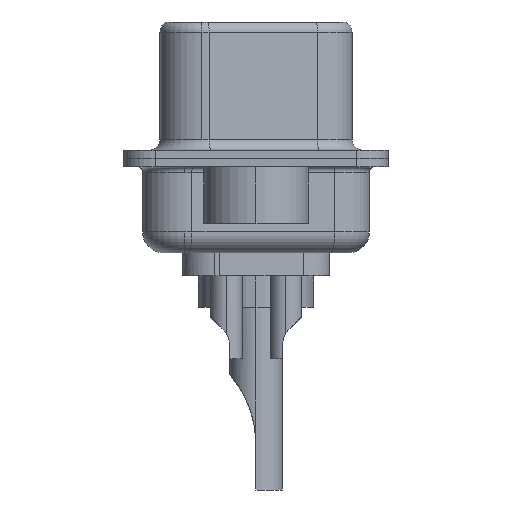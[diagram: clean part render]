
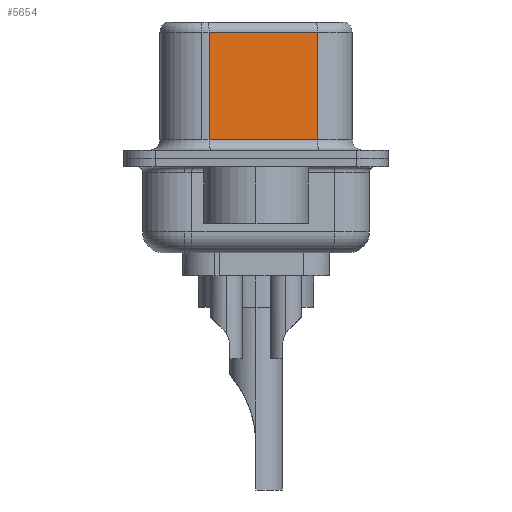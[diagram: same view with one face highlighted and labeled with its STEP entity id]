
A CAD part, left-side view. The second image highlights one B-rep face of the part: STEP entity #5654.
In plain terms, the highlighted planar face has unit normal (-0.985, -0.174, 0).
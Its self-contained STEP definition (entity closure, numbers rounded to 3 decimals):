
#146 = VERTEX_POINT ( 'NONE', #6224 ) ;
#476 = ORIENTED_EDGE ( 'NONE', *, *, #2638, .T. ) ;
#1671 = EDGE_CURVE ( 'NONE', #14607, #146, #11014, .T. ) ;
#1819 = CARTESIAN_POINT ( 'NONE',  ( 4.565, -2.927, 6.52 ) ) ;
#2638 = EDGE_CURVE ( 'NONE', #146, #15769, #15951, .T. ) ;
#3247 = DIRECTION ( 'NONE',  ( -0.174, 0.985, 0. ) ) ;
#3929 = LINE ( 'NONE', #13872, #10312 ) ;
#4091 = CARTESIAN_POINT ( 'NONE',  ( 4.565, -2.927, 0.9 ) ) ;
#4620 = DIRECTION ( 'NONE',  ( 0.174, -0.985, 0. ) ) ;
#5042 = CARTESIAN_POINT ( 'NONE',  ( 4.565, -2.927, 6.02 ) ) ;
#5441 = VECTOR ( 'NONE', #9369, 1000. ) ;
#5654 = ADVANCED_FACE ( 'NONE', ( #14398 ), #15184, .F. ) ;
#6224 = CARTESIAN_POINT ( 'NONE',  ( 3.655, 2.233, 6.02 ) ) ;
#6490 = DIRECTION ( 'NONE',  ( -0.174, 0.985, 0. ) ) ;
#7057 = ORIENTED_EDGE ( 'NONE', *, *, #7170, .F. ) ;
#7162 = LINE ( 'NONE', #16521, #11160 ) ;
#7170 = EDGE_CURVE ( 'NONE', #14607, #16997, #7162, .T. ) ;
#7173 = EDGE_CURVE ( 'NONE', #15769, #16997, #3929, .T. ) ;
#7406 = VECTOR ( 'NONE', #6490, 1000. ) ;
#7483 = ORIENTED_EDGE ( 'NONE', *, *, #1671, .T. ) ;
#8137 = CARTESIAN_POINT ( 'NONE',  ( 3.655, 2.233, 0.9 ) ) ;
#8695 = DIRECTION ( 'NONE',  ( 0., 0., -1. ) ) ;
#9369 = DIRECTION ( 'NONE',  ( 0., 0., -1. ) ) ;
#10312 = VECTOR ( 'NONE', #4620, 1000. ) ;
#10691 = CARTESIAN_POINT ( 'NONE',  ( 4.565, -2.927, 6.02 ) ) ;
#10795 = EDGE_LOOP ( 'NONE', ( #7057, #7483, #476, #11469 ) ) ;
#11014 = LINE ( 'NONE', #5042, #7406 ) ;
#11160 = VECTOR ( 'NONE', #8695, 1000. ) ;
#11429 = DIRECTION ( 'NONE',  ( 0.985, 0.174, 0. ) ) ;
#11469 = ORIENTED_EDGE ( 'NONE', *, *, #7173, .T. ) ;
#13872 = CARTESIAN_POINT ( 'NONE',  ( 4.565, -2.927, 0.9 ) ) ;
#14173 = CARTESIAN_POINT ( 'NONE',  ( 3.655, 2.233, 6.52 ) ) ;
#14398 = FACE_OUTER_BOUND ( 'NONE', #10795, .T. ) ;
#14607 = VERTEX_POINT ( 'NONE', #10691 ) ;
#15184 = PLANE ( 'NONE',  #15253 ) ;
#15253 = AXIS2_PLACEMENT_3D ( 'NONE', #1819, #11429, #3247 ) ;
#15769 = VERTEX_POINT ( 'NONE', #8137 ) ;
#15951 = LINE ( 'NONE', #14173, #5441 ) ;
#16521 = CARTESIAN_POINT ( 'NONE',  ( 4.565, -2.927, 6.52 ) ) ;
#16997 = VERTEX_POINT ( 'NONE', #4091 ) ;
